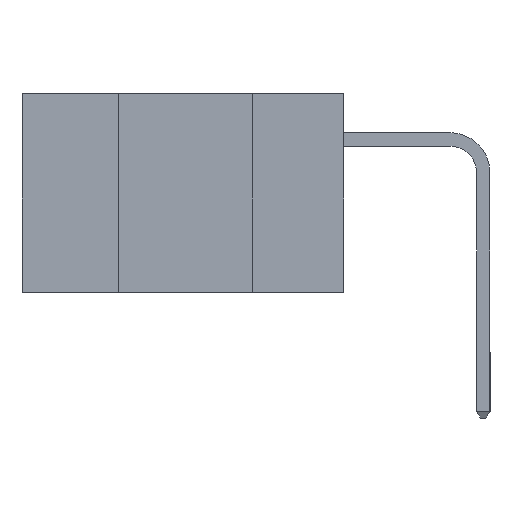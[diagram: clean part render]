
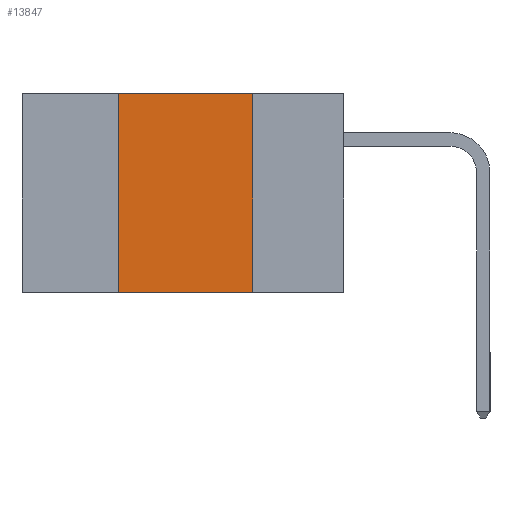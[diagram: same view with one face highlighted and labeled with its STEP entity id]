
A CAD part, left-side view. The second image highlights one B-rep face of the part: STEP entity #13847.
In plain terms, the highlighted planar face has unit normal (-1, 0, 0).
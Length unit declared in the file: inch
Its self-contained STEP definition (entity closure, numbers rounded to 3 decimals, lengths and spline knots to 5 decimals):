
#499 = CARTESIAN_POINT ( 'NONE',  ( 0., 0.17, 0. ) ) ;
#1255 = ORIENTED_EDGE ( 'NONE', *, *, #21414, .T. ) ;
#1632 = CARTESIAN_POINT ( 'NONE',  ( 0., 0.42, -0.37 ) ) ;
#2380 = EDGE_LOOP ( 'NONE', ( #18000, #13350, #5197, #1255 ) ) ;
#2552 = VERTEX_POINT ( 'NONE', #4839 ) ;
#2555 = CARTESIAN_POINT ( 'NONE',  ( 0., 0.6, 0. ) ) ;
#2573 = CARTESIAN_POINT ( 'NONE',  ( 0., 0.6, -0.37 ) ) ;
#2902 = EDGE_CURVE ( 'NONE', #13516, #3454, #22396, .T. ) ;
#3454 = VERTEX_POINT ( 'NONE', #18401 ) ;
#4183 = DIRECTION ( 'NONE',  ( 1., 0., 0. ) ) ;
#4539 = DIRECTION ( 'NONE',  ( 0., 0., -1. ) ) ;
#4642 = DIRECTION ( 'NONE',  ( 0., -1., 0. ) ) ;
#4839 = CARTESIAN_POINT ( 'NONE',  ( 0., 0.17, 0. ) ) ;
#5197 = ORIENTED_EDGE ( 'NONE', *, *, #2902, .F. ) ;
#6716 = LINE ( 'NONE', #18151, #21601 ) ;
#8345 = VERTEX_POINT ( 'NONE', #9340 ) ;
#9340 = CARTESIAN_POINT ( 'NONE',  ( 0., 0.17, -0.37 ) ) ;
#10846 = DIRECTION ( 'NONE',  ( 0., 0., 1. ) ) ;
#12268 = CARTESIAN_POINT ( 'NONE',  ( 0., 0.42, 0. ) ) ;
#12415 = LINE ( 'NONE', #499, #21503 ) ;
#13350 = ORIENTED_EDGE ( 'NONE', *, *, #19971, .F. ) ;
#13516 = VERTEX_POINT ( 'NONE', #1632 ) ;
#13847 = ADVANCED_FACE ( 'NONE', ( #16572 ), #14224, .F. ) ;
#14224 = PLANE ( 'NONE',  #21939 ) ;
#15730 = VECTOR ( 'NONE', #10846, 39.37008 ) ;
#16202 = VECTOR ( 'NONE', #16531, 39.37008 ) ;
#16531 = DIRECTION ( 'NONE',  ( 0., -1., 0. ) ) ;
#16572 = FACE_OUTER_BOUND ( 'NONE', #2380, .T. ) ;
#17141 = LINE ( 'NONE', #2573, #16202 ) ;
#18000 = ORIENTED_EDGE ( 'NONE', *, *, #25225, .F. ) ;
#18094 = DIRECTION ( 'NONE',  ( 0., 0., -1. ) ) ;
#18151 = CARTESIAN_POINT ( 'NONE',  ( 0., 0.6, 0. ) ) ;
#18401 = CARTESIAN_POINT ( 'NONE',  ( 0., 0.42, 0. ) ) ;
#19971 = EDGE_CURVE ( 'NONE', #3454, #2552, #6716, .T. ) ;
#21414 = EDGE_CURVE ( 'NONE', #13516, #8345, #17141, .T. ) ;
#21503 = VECTOR ( 'NONE', #18094, 39.37008 ) ;
#21601 = VECTOR ( 'NONE', #4642, 39.37008 ) ;
#21939 = AXIS2_PLACEMENT_3D ( 'NONE', #2555, #4183, #4539 ) ;
#22396 = LINE ( 'NONE', #12268, #15730 ) ;
#25225 = EDGE_CURVE ( 'NONE', #2552, #8345, #12415, .T. ) ;
